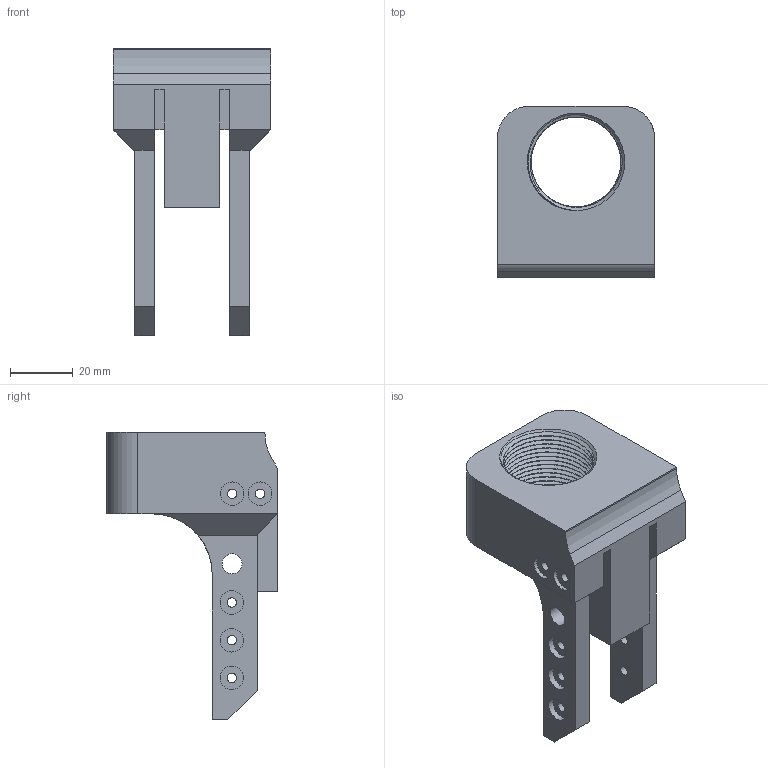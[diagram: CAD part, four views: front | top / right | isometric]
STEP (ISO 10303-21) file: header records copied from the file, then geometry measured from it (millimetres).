
FILE_DESCRIPTION (( 'STEP AP214' ), '1' );
FILE_NAME ('No_Safety_Reinforced_Buffer.step', '2016-01-30T20:06:10', ( 'WarFairy' ), ( '' ), 'SwSTEP 2.0', 'SolidWorks 2015', '' );
FILE_SCHEMA (( 'AUTOMOTIVE_DESIGN' ));
Length unit declared in the file: millimetre
Products named in the file (1): No_Safety_Reinforced_Buffer
Bounding box: 50 x 54.46 x 91.53 mm (x, y, z)
Volume: 71185.1 mm3; surface area: 22905.7 mm2
Topology: 1 solids, 1 shells, 158 faces, 446 edges, 299 vertices
Faces by surface type: plane 62, cylinder 52, bspline 42, cone 2
Full cylindrical faces by diameter (mm): 3 x12, 6.35 x4, 6.477 x1, 7.5 x8
Entity records: 43178 total; most frequent: CARTESIAN_POINT 39665, ORIENTED_EDGE 816, DIRECTION 532, EDGE_CURVE 408, VERTEX_POINT 287, EDGE_LOOP 227, AXIS2_PLACEMENT_3D 189, FACE_OUTER_BOUND 183
